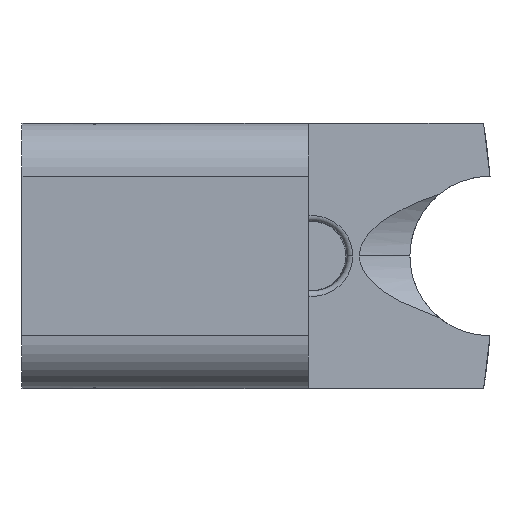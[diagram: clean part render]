
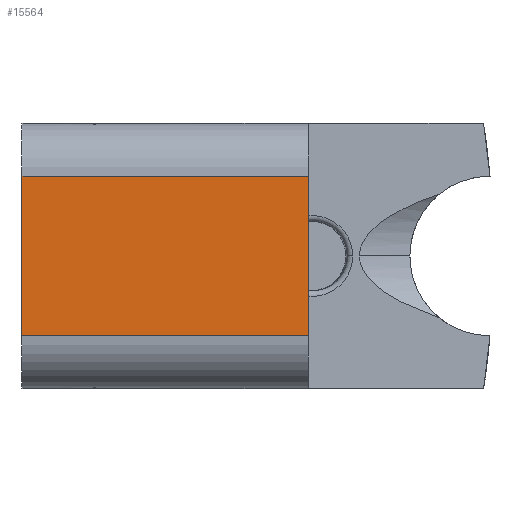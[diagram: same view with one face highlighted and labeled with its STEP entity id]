
A CAD part, left-side view. The second image highlights one B-rep face of the part: STEP entity #15564.
In plain terms, the highlighted planar face has unit normal (-1, 0, 0).
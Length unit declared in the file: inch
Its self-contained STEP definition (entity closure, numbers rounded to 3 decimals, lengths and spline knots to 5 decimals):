
#638 = PLANE ( 'NONE',  #11932 ) ;
#1178 = DIRECTION ( 'NONE',  ( 0., 0., -1. ) ) ;
#1237 = CARTESIAN_POINT ( 'NONE',  ( 0., 0., 0. ) ) ;
#1378 = VECTOR ( 'NONE', #1178, 39.37008 ) ;
#1652 = EDGE_CURVE ( 'NONE', #7555, #4343, #13440, .T. ) ;
#2088 = VECTOR ( 'NONE', #6050, 39.37008 ) ;
#3141 = ORIENTED_EDGE ( 'NONE', *, *, #4718, .T. ) ;
#4046 = LINE ( 'NONE', #12016, #10623 ) ;
#4343 = VERTEX_POINT ( 'NONE', #4915 ) ;
#4391 = VERTEX_POINT ( 'NONE', #6143 ) ;
#4622 = DIRECTION ( 'NONE',  ( 0., -1., 0. ) ) ;
#4718 = EDGE_CURVE ( 'NONE', #4391, #4343, #10920, .T. ) ;
#4915 = CARTESIAN_POINT ( 'NONE',  ( 0., 1.347, 0.375 ) ) ;
#5599 = DIRECTION ( 'NONE',  ( 0., 0., 1. ) ) ;
#6050 = DIRECTION ( 'NONE',  ( 0., 0., 1. ) ) ;
#6143 = CARTESIAN_POINT ( 'NONE',  ( 0., 0., 0.375 ) ) ;
#6734 = CARTESIAN_POINT ( 'NONE',  ( 0., 0., -0.375 ) ) ;
#7555 = VERTEX_POINT ( 'NONE', #8121 ) ;
#8037 = ORIENTED_EDGE ( 'NONE', *, *, #10472, .F. ) ;
#8054 = VECTOR ( 'NONE', #14243, 39.37008 ) ;
#8121 = CARTESIAN_POINT ( 'NONE',  ( 0., 1.347, -0.375 ) ) ;
#8167 = ORIENTED_EDGE ( 'NONE', *, *, #12729, .T. ) ;
#8195 = ORIENTED_EDGE ( 'NONE', *, *, #1652, .F. ) ;
#10163 = CARTESIAN_POINT ( 'NONE',  ( 0., 1.347, -0.375 ) ) ;
#10472 = EDGE_CURVE ( 'NONE', #4391, #15069, #13710, .T. ) ;
#10623 = VECTOR ( 'NONE', #4622, 39.37008 ) ;
#10920 = LINE ( 'NONE', #15501, #8054 ) ;
#11932 = AXIS2_PLACEMENT_3D ( 'NONE', #6734, #12979, #5599 ) ;
#12016 = CARTESIAN_POINT ( 'NONE',  ( 0., 0.52115, -0.375 ) ) ;
#12315 = FACE_OUTER_BOUND ( 'NONE', #14588, .T. ) ;
#12729 = EDGE_CURVE ( 'NONE', #7555, #15069, #4046, .T. ) ;
#12979 = DIRECTION ( 'NONE',  ( -1., 0., 0. ) ) ;
#13440 = LINE ( 'NONE', #10163, #2088 ) ;
#13710 = LINE ( 'NONE', #1237, #1378 ) ;
#14243 = DIRECTION ( 'NONE',  ( 0., 1., 0. ) ) ;
#14588 = EDGE_LOOP ( 'NONE', ( #8167, #8037, #3141, #8195 ) ) ;
#14992 = CARTESIAN_POINT ( 'NONE',  ( 0., 0., -0.375 ) ) ;
#15069 = VERTEX_POINT ( 'NONE', #14992 ) ;
#15501 = CARTESIAN_POINT ( 'NONE',  ( 0., 0.52115, 0.375 ) ) ;
#15564 = ADVANCED_FACE ( 'NONE', ( #12315 ), #638, .T. ) ;
